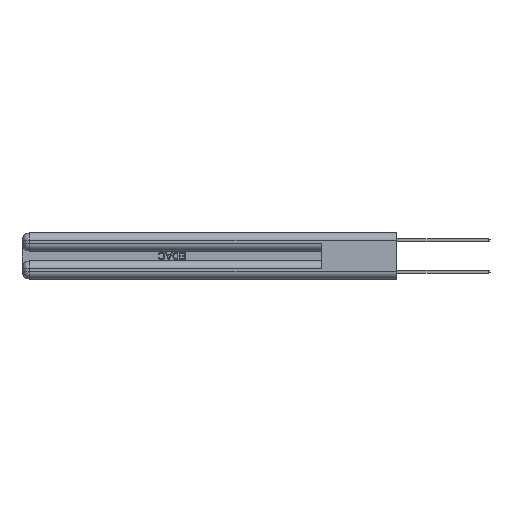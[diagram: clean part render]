
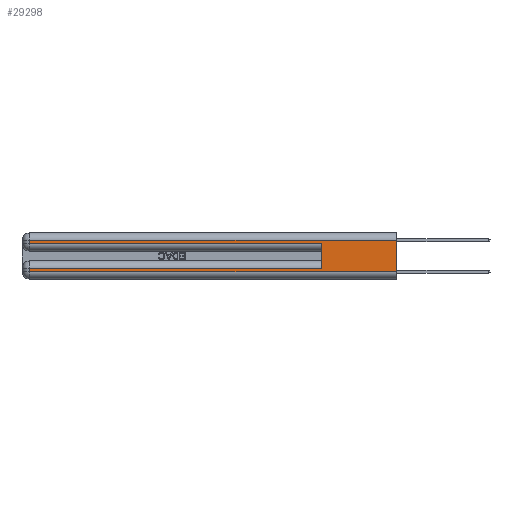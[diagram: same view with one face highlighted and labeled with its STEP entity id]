
A CAD part, left-side view. The second image highlights one B-rep face of the part: STEP entity #29298.
In plain terms, the highlighted planar face has unit normal (-1, 0, 0).
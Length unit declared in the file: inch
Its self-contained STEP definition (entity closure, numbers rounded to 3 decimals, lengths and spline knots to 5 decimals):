
#441 = CARTESIAN_POINT ( 'NONE',  ( 0., 0., 0.06 ) ) ;
#1187 = VERTEX_POINT ( 'NONE', #5897 ) ;
#1422 = EDGE_CURVE ( 'NONE', #34234, #12077, #28141, .T. ) ;
#1694 = CARTESIAN_POINT ( 'NONE',  ( 0., 2.94, 0.085 ) ) ;
#1763 = CARTESIAN_POINT ( 'NONE',  ( 0., 0.6, 0.285 ) ) ;
#1771 = LINE ( 'NONE', #6923, #25902 ) ;
#1781 = CARTESIAN_POINT ( 'NONE',  ( 0., 2.94, 0.06 ) ) ;
#1797 = LINE ( 'NONE', #9454, #2721 ) ;
#2100 = VECTOR ( 'NONE', #21446, 39.37008 ) ;
#2321 = CARTESIAN_POINT ( 'NONE',  ( 0., 2.94, 0.285 ) ) ;
#2590 = ORIENTED_EDGE ( 'NONE', *, *, #24932, .T. ) ;
#2721 = VECTOR ( 'NONE', #25826, 39.37008 ) ;
#3382 = ORIENTED_EDGE ( 'NONE', *, *, #18997, .T. ) ;
#4625 = DIRECTION ( 'NONE',  ( 0., 1., 0. ) ) ;
#5162 = CARTESIAN_POINT ( 'NONE',  ( 0., 2.94, 0.31 ) ) ;
#5897 = CARTESIAN_POINT ( 'NONE',  ( 0., 0.6, 0.085 ) ) ;
#6923 = CARTESIAN_POINT ( 'NONE',  ( 0., 0., 0.31 ) ) ;
#7083 = VERTEX_POINT ( 'NONE', #5162 ) ;
#7758 = CARTESIAN_POINT ( 'NONE',  ( 0., 0.6, 0.145 ) ) ;
#8207 = LINE ( 'NONE', #14239, #15999 ) ;
#9454 = CARTESIAN_POINT ( 'NONE',  ( 0., 0., 0.37 ) ) ;
#11102 = PLANE ( 'NONE',  #25723 ) ;
#11306 = ORIENTED_EDGE ( 'NONE', *, *, #19013, .T. ) ;
#12077 = VERTEX_POINT ( 'NONE', #1763 ) ;
#12105 = CARTESIAN_POINT ( 'NONE',  ( 0., 0., 0.285 ) ) ;
#13427 = VERTEX_POINT ( 'NONE', #29184 ) ;
#13898 = EDGE_CURVE ( 'NONE', #1187, #12077, #21794, .T. ) ;
#14122 = DIRECTION ( 'NONE',  ( 0., 0., -1. ) ) ;
#14173 = VERTEX_POINT ( 'NONE', #1694 ) ;
#14239 = CARTESIAN_POINT ( 'NONE',  ( 0., 0., 0.085 ) ) ;
#14650 = EDGE_LOOP ( 'NONE', ( #20221, #3382, #11306, #16140, #24464, #17411, #2590, #34959 ) ) ;
#15829 = EDGE_CURVE ( 'NONE', #18509, #13427, #1797, .T. ) ;
#15999 = VECTOR ( 'NONE', #19048, 39.37008 ) ;
#16140 = ORIENTED_EDGE ( 'NONE', *, *, #1422, .T. ) ;
#16627 = DIRECTION ( 'NONE',  ( 0., -1., 0. ) ) ;
#17151 = CARTESIAN_POINT ( 'NONE',  ( 0., 2.94, 0.37 ) ) ;
#17411 = ORIENTED_EDGE ( 'NONE', *, *, #28496, .T. ) ;
#17515 = DIRECTION ( 'NONE',  ( 0., 0., -1. ) ) ;
#18476 = DIRECTION ( 'NONE',  ( 0., 0., -1. ) ) ;
#18509 = VERTEX_POINT ( 'NONE', #26728 ) ;
#18997 = EDGE_CURVE ( 'NONE', #18509, #7083, #1771, .T. ) ;
#19013 = EDGE_CURVE ( 'NONE', #7083, #34234, #26330, .T. ) ;
#19048 = DIRECTION ( 'NONE',  ( 0., 1., 0. ) ) ;
#19282 = FACE_OUTER_BOUND ( 'NONE', #14650, .T. ) ;
#19637 = VECTOR ( 'NONE', #18476, 39.37008 ) ;
#20221 = ORIENTED_EDGE ( 'NONE', *, *, #15829, .F. ) ;
#21446 = DIRECTION ( 'NONE',  ( 0., 0., 1. ) ) ;
#21794 = LINE ( 'NONE', #7758, #2100 ) ;
#22142 = LINE ( 'NONE', #441, #24892 ) ;
#23432 = EDGE_CURVE ( 'NONE', #28735, #13427, #22142, .T. ) ;
#24464 = ORIENTED_EDGE ( 'NONE', *, *, #13898, .F. ) ;
#24892 = VECTOR ( 'NONE', #16627, 39.37008 ) ;
#24932 = EDGE_CURVE ( 'NONE', #14173, #28735, #30697, .T. ) ;
#25723 = AXIS2_PLACEMENT_3D ( 'NONE', #30666, #27307, #14122 ) ;
#25826 = DIRECTION ( 'NONE',  ( 0., 0., -1. ) ) ;
#25902 = VECTOR ( 'NONE', #4625, 39.37008 ) ;
#26330 = LINE ( 'NONE', #34665, #19637 ) ;
#26728 = CARTESIAN_POINT ( 'NONE',  ( 0., 0., 0.31 ) ) ;
#27307 = DIRECTION ( 'NONE',  ( 1., 0., 0. ) ) ;
#28141 = LINE ( 'NONE', #12105, #32624 ) ;
#28496 = EDGE_CURVE ( 'NONE', #1187, #14173, #8207, .T. ) ;
#28735 = VERTEX_POINT ( 'NONE', #1781 ) ;
#29184 = CARTESIAN_POINT ( 'NONE',  ( 0., 0., 0.06 ) ) ;
#29298 = ADVANCED_FACE ( 'NONE', ( #19282 ), #11102, .F. ) ;
#30457 = DIRECTION ( 'NONE',  ( 0., -1., 0. ) ) ;
#30630 = VECTOR ( 'NONE', #17515, 39.37008 ) ;
#30666 = CARTESIAN_POINT ( 'NONE',  ( 0., 0., 0.37 ) ) ;
#30697 = LINE ( 'NONE', #17151, #30630 ) ;
#32624 = VECTOR ( 'NONE', #30457, 39.37008 ) ;
#34234 = VERTEX_POINT ( 'NONE', #2321 ) ;
#34665 = CARTESIAN_POINT ( 'NONE',  ( 0., 2.94, 0.37 ) ) ;
#34959 = ORIENTED_EDGE ( 'NONE', *, *, #23432, .T. ) ;
